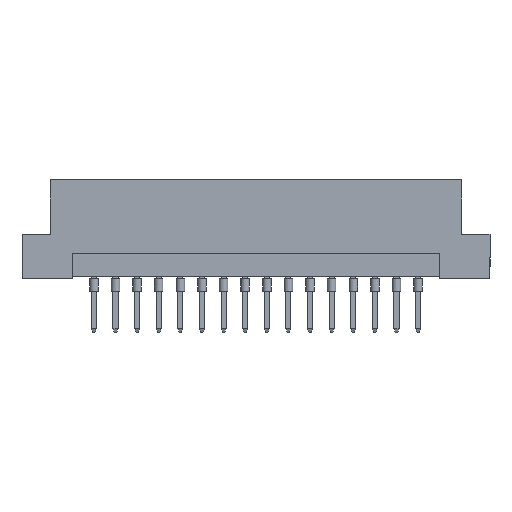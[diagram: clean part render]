
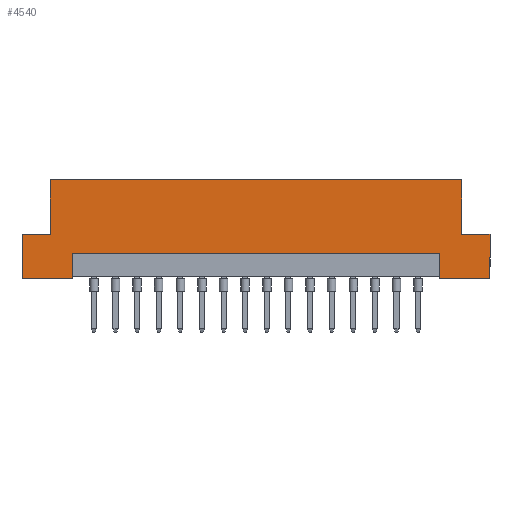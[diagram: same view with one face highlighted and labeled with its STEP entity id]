
A CAD part, front view. The second image highlights one B-rep face of the part: STEP entity #4540.
In plain terms, the highlighted planar face has unit normal (0, -1, 0).
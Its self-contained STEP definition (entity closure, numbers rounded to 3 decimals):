
#18 = CARTESIAN_POINT ( 'NONE',  ( 21.6, -4.3, 3. ) ) ;
#60 = EDGE_CURVE ( 'NONE', #7220, #4230, #3040, .T. ) ;
#88 = DIRECTION ( 'NONE',  ( 0., 0., 1. ) ) ;
#95 = ORIENTED_EDGE ( 'NONE', *, *, #7019, .T. ) ;
#169 = PLANE ( 'NONE',  #5712 ) ;
#179 = DIRECTION ( 'NONE',  ( 1., 0., 0. ) ) ;
#282 = ORIENTED_EDGE ( 'NONE', *, *, #5659, .F. ) ;
#292 = CARTESIAN_POINT ( 'NONE',  ( -21.6, -4.3, 3. ) ) ;
#297 = CARTESIAN_POINT ( 'NONE',  ( 21.6, -4.3, 0.2 ) ) ;
#304 = ORIENTED_EDGE ( 'NONE', *, *, #60, .T. ) ;
#424 = CARTESIAN_POINT ( 'NONE',  ( -24.2, -4.3, 5.2 ) ) ;
#645 = VERTEX_POINT ( 'NONE', #424 ) ;
#697 = ORIENTED_EDGE ( 'NONE', *, *, #2195, .T. ) ;
#706 = FACE_OUTER_BOUND ( 'NONE', #5796, .T. ) ;
#752 = DIRECTION ( 'NONE',  ( -1., 0., 0. ) ) ;
#933 = VERTEX_POINT ( 'NONE', #5543 ) ;
#1033 = DIRECTION ( 'NONE',  ( 0., 0., 1. ) ) ;
#1313 = CARTESIAN_POINT ( 'NONE',  ( -27.5, -4.3, 5.2 ) ) ;
#1417 = VERTEX_POINT ( 'NONE', #3735 ) ;
#1484 = DIRECTION ( 'NONE',  ( 0., 0., -1. ) ) ;
#1514 = CARTESIAN_POINT ( 'NONE',  ( 27.5, -4.3, 5.2 ) ) ;
#1537 = VERTEX_POINT ( 'NONE', #292 ) ;
#1660 = CARTESIAN_POINT ( 'NONE',  ( 27.5, -4.3, 0. ) ) ;
#1714 = VECTOR ( 'NONE', #5704, 1000. ) ;
#1733 = ORIENTED_EDGE ( 'NONE', *, *, #3045, .F. ) ;
#1815 = VERTEX_POINT ( 'NONE', #7258 ) ;
#1954 = LINE ( 'NONE', #3882, #4606 ) ;
#2088 = VECTOR ( 'NONE', #5250, 1000. ) ;
#2131 = LINE ( 'NONE', #6433, #1714 ) ;
#2155 = EDGE_CURVE ( 'NONE', #2475, #5036, #2131, .T. ) ;
#2195 = EDGE_CURVE ( 'NONE', #933, #6926, #2200, .T. ) ;
#2200 = LINE ( 'NONE', #1660, #3836 ) ;
#2254 = LINE ( 'NONE', #3543, #2088 ) ;
#2435 = CARTESIAN_POINT ( 'NONE',  ( 27.5, -4.3, 11.6 ) ) ;
#2475 = VERTEX_POINT ( 'NONE', #7438 ) ;
#2564 = CARTESIAN_POINT ( 'NONE',  ( 24.2, -4.3, 11.6 ) ) ;
#2917 = LINE ( 'NONE', #6952, #6467 ) ;
#3040 = LINE ( 'NONE', #5439, #5779 ) ;
#3045 = EDGE_CURVE ( 'NONE', #1815, #645, #6700, .T. ) ;
#3069 = ORIENTED_EDGE ( 'NONE', *, *, #6069, .F. ) ;
#3373 = VERTEX_POINT ( 'NONE', #18 ) ;
#3543 = CARTESIAN_POINT ( 'NONE',  ( -27.5, -4.3, 11.6 ) ) ;
#3580 = DIRECTION ( 'NONE',  ( 0., 1., 0. ) ) ;
#3602 = CARTESIAN_POINT ( 'NONE',  ( 27.5, -4.3, 0. ) ) ;
#3735 = CARTESIAN_POINT ( 'NONE',  ( 27.5, -4.3, 5.2 ) ) ;
#3817 = LINE ( 'NONE', #297, #5353 ) ;
#3836 = VECTOR ( 'NONE', #4602, 1000. ) ;
#3882 = CARTESIAN_POINT ( 'NONE',  ( -21.6, -4.3, 3. ) ) ;
#3938 = CARTESIAN_POINT ( 'NONE',  ( 27.5, -4.3, 11.6 ) ) ;
#4029 = LINE ( 'NONE', #1514, #7197 ) ;
#4094 = ORIENTED_EDGE ( 'NONE', *, *, #2155, .T. ) ;
#4230 = VERTEX_POINT ( 'NONE', #2564 ) ;
#4244 = CARTESIAN_POINT ( 'NONE',  ( -24.2, -4.3, 11.6 ) ) ;
#4294 = ORIENTED_EDGE ( 'NONE', *, *, #7588, .F. ) ;
#4397 = CARTESIAN_POINT ( 'NONE',  ( -21.6, -4.3, 0. ) ) ;
#4494 = LINE ( 'NONE', #5592, #6476 ) ;
#4540 = ADVANCED_FACE ( 'NONE', ( #706 ), #169, .F. ) ;
#4602 = DIRECTION ( 'NONE',  ( 1., 0., 0. ) ) ;
#4606 = VECTOR ( 'NONE', #7435, 1000. ) ;
#4965 = DIRECTION ( 'NONE',  ( 0., 0., -1. ) ) ;
#5036 = VERTEX_POINT ( 'NONE', #4397 ) ;
#5217 = EDGE_CURVE ( 'NONE', #7220, #1417, #4029, .T. ) ;
#5250 = DIRECTION ( 'NONE',  ( 0., 0., -1. ) ) ;
#5353 = VECTOR ( 'NONE', #6841, 1000. ) ;
#5439 = CARTESIAN_POINT ( 'NONE',  ( 24.2, -4.3, 5.2 ) ) ;
#5475 = VECTOR ( 'NONE', #7512, 1000. ) ;
#5543 = CARTESIAN_POINT ( 'NONE',  ( 21.6, -4.3, 0. ) ) ;
#5558 = CARTESIAN_POINT ( 'NONE',  ( -21.6, -4.3, 0.2 ) ) ;
#5592 = CARTESIAN_POINT ( 'NONE',  ( 27.5, -4.3, 11.6 ) ) ;
#5659 = EDGE_CURVE ( 'NONE', #933, #3373, #3817, .T. ) ;
#5683 = ORIENTED_EDGE ( 'NONE', *, *, #5821, .F. ) ;
#5704 = DIRECTION ( 'NONE',  ( 1., 0., 0. ) ) ;
#5712 = AXIS2_PLACEMENT_3D ( 'NONE', #2435, #3580, #752 ) ;
#5739 = DIRECTION ( 'NONE',  ( 1., 0., 0. ) ) ;
#5747 = EDGE_CURVE ( 'NONE', #1815, #2475, #2254, .T. ) ;
#5779 = VECTOR ( 'NONE', #88, 1000. ) ;
#5796 = EDGE_LOOP ( 'NONE', ( #95, #282, #697, #7080, #6557, #304, #4294, #5683, #1733, #7267, #4094, #3069 ) ) ;
#5821 = EDGE_CURVE ( 'NONE', #645, #5907, #2917, .T. ) ;
#5907 = VERTEX_POINT ( 'NONE', #4244 ) ;
#6069 = EDGE_CURVE ( 'NONE', #1537, #5036, #6294, .T. ) ;
#6161 = EDGE_CURVE ( 'NONE', #1417, #6926, #4494, .T. ) ;
#6294 = LINE ( 'NONE', #5558, #7585 ) ;
#6348 = VECTOR ( 'NONE', #179, 1000. ) ;
#6354 = CARTESIAN_POINT ( 'NONE',  ( 24.2, -4.3, 5.2 ) ) ;
#6433 = CARTESIAN_POINT ( 'NONE',  ( 27.5, -4.3, 0. ) ) ;
#6467 = VECTOR ( 'NONE', #1033, 1000. ) ;
#6476 = VECTOR ( 'NONE', #4965, 1000. ) ;
#6557 = ORIENTED_EDGE ( 'NONE', *, *, #5217, .F. ) ;
#6700 = LINE ( 'NONE', #1313, #6348 ) ;
#6841 = DIRECTION ( 'NONE',  ( 0., 0., 1. ) ) ;
#6926 = VERTEX_POINT ( 'NONE', #3602 ) ;
#6952 = CARTESIAN_POINT ( 'NONE',  ( -24.2, -4.3, 5.2 ) ) ;
#7019 = EDGE_CURVE ( 'NONE', #1537, #3373, #1954, .T. ) ;
#7080 = ORIENTED_EDGE ( 'NONE', *, *, #6161, .F. ) ;
#7197 = VECTOR ( 'NONE', #5739, 1000. ) ;
#7220 = VERTEX_POINT ( 'NONE', #6354 ) ;
#7258 = CARTESIAN_POINT ( 'NONE',  ( -27.5, -4.3, 5.2 ) ) ;
#7267 = ORIENTED_EDGE ( 'NONE', *, *, #5747, .T. ) ;
#7428 = LINE ( 'NONE', #3938, #5475 ) ;
#7435 = DIRECTION ( 'NONE',  ( 1., 0., 0. ) ) ;
#7438 = CARTESIAN_POINT ( 'NONE',  ( -27.5, -4.3, 0. ) ) ;
#7512 = DIRECTION ( 'NONE',  ( 1., 0., 0. ) ) ;
#7585 = VECTOR ( 'NONE', #1484, 1000. ) ;
#7588 = EDGE_CURVE ( 'NONE', #5907, #4230, #7428, .T. ) ;
